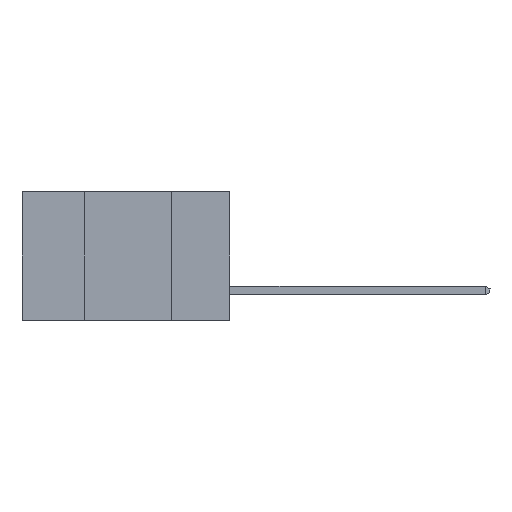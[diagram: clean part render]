
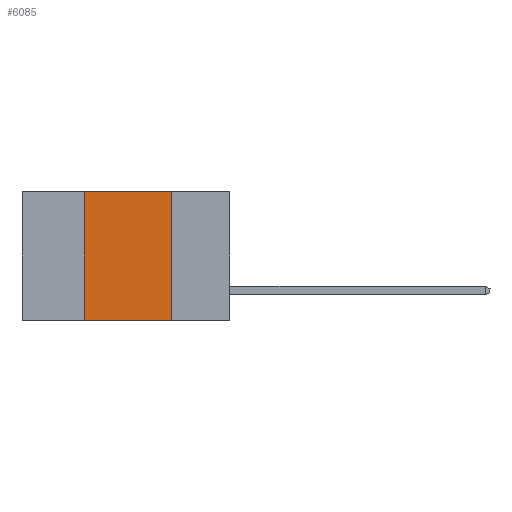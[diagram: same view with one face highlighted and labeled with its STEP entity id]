
A CAD part, left-side view. The second image highlights one B-rep face of the part: STEP entity #6085.
In plain terms, the highlighted planar face has unit normal (-1, 0, 0).
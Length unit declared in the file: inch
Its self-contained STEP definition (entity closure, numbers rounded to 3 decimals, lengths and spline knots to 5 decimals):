
#998 = LINE ( 'NONE', #11783, #14339 ) ;
#1652 = AXIS2_PLACEMENT_3D ( 'NONE', #17259, #21110, #15455 ) ;
#2280 = CARTESIAN_POINT ( 'NONE',  ( 0., 0.17, 0. ) ) ;
#2528 = CARTESIAN_POINT ( 'NONE',  ( 0., 0.42, 0. ) ) ;
#2859 = PLANE ( 'NONE',  #1652 ) ;
#2871 = CARTESIAN_POINT ( 'NONE',  ( 0., 0.17, -0.37 ) ) ;
#2976 = FACE_OUTER_BOUND ( 'NONE', #4132, .T. ) ;
#3156 = CARTESIAN_POINT ( 'NONE',  ( 0., 0.6, 0. ) ) ;
#4132 = EDGE_LOOP ( 'NONE', ( #15827, #8958, #11343, #12115 ) ) ;
#5469 = VECTOR ( 'NONE', #12418, 39.37008 ) ;
#5777 = VECTOR ( 'NONE', #6726, 39.37008 ) ;
#6085 = ADVANCED_FACE ( 'NONE', ( #2976 ), #2859, .F. ) ;
#6726 = DIRECTION ( 'NONE',  ( 0., -1., 0. ) ) ;
#8184 = LINE ( 'NONE', #10202, #5777 ) ;
#8367 = VERTEX_POINT ( 'NONE', #22502 ) ;
#8535 = EDGE_CURVE ( 'NONE', #8367, #21278, #8184, .T. ) ;
#8958 = ORIENTED_EDGE ( 'NONE', *, *, #20894, .F. ) ;
#9269 = VERTEX_POINT ( 'NONE', #2280 ) ;
#9359 = DIRECTION ( 'NONE',  ( 0., -1., 0. ) ) ;
#10202 = CARTESIAN_POINT ( 'NONE',  ( 0., 0.6, -0.37 ) ) ;
#11023 = LINE ( 'NONE', #3156, #15096 ) ;
#11343 = ORIENTED_EDGE ( 'NONE', *, *, #22189, .F. ) ;
#11783 = CARTESIAN_POINT ( 'NONE',  ( 0., 0.42, -0.37 ) ) ;
#12115 = ORIENTED_EDGE ( 'NONE', *, *, #8535, .T. ) ;
#12293 = CARTESIAN_POINT ( 'NONE',  ( 0., 0.17, -0.37 ) ) ;
#12418 = DIRECTION ( 'NONE',  ( 0., 0., -1. ) ) ;
#14339 = VECTOR ( 'NONE', #15516, 39.37008 ) ;
#15096 = VECTOR ( 'NONE', #9359, 39.37008 ) ;
#15455 = DIRECTION ( 'NONE',  ( 0., 0., -1. ) ) ;
#15516 = DIRECTION ( 'NONE',  ( 0., 0., 1. ) ) ;
#15827 = ORIENTED_EDGE ( 'NONE', *, *, #19374, .F. ) ;
#17259 = CARTESIAN_POINT ( 'NONE',  ( 0., 0.6, 0. ) ) ;
#19374 = EDGE_CURVE ( 'NONE', #9269, #21278, #19779, .T. ) ;
#19779 = LINE ( 'NONE', #12293, #5469 ) ;
#20894 = EDGE_CURVE ( 'NONE', #21128, #9269, #11023, .T. ) ;
#21110 = DIRECTION ( 'NONE',  ( 1., 0., 0. ) ) ;
#21128 = VERTEX_POINT ( 'NONE', #2528 ) ;
#21278 = VERTEX_POINT ( 'NONE', #2871 ) ;
#22189 = EDGE_CURVE ( 'NONE', #8367, #21128, #998, .T. ) ;
#22502 = CARTESIAN_POINT ( 'NONE',  ( 0., 0.42, -0.37 ) ) ;
